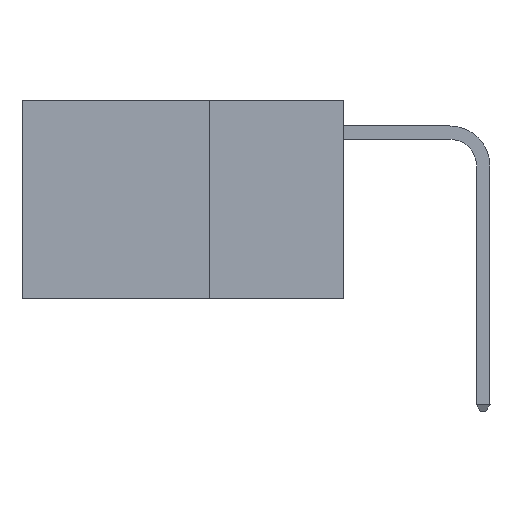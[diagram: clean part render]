
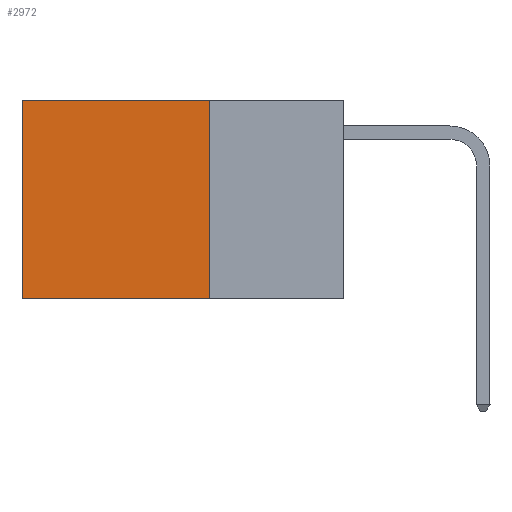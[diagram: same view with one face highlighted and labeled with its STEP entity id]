
A CAD part, left-side view. The second image highlights one B-rep face of the part: STEP entity #2972.
In plain terms, the highlighted planar face has unit normal (-1, 0, 0).
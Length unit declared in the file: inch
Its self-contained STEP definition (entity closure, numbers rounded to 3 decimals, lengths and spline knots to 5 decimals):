
#190 = ORIENTED_EDGE ( 'NONE', *, *, #12204, .T. ) ;
#809 = CARTESIAN_POINT ( 'NONE',  ( 0.2625, 0.25, 0. ) ) ;
#930 = VERTEX_POINT ( 'NONE', #4951 ) ;
#1069 = EDGE_CURVE ( 'NONE', #10929, #2018, #9868, .T. ) ;
#1940 = DIRECTION ( 'NONE',  ( 0., 0., -1. ) ) ;
#2018 = VERTEX_POINT ( 'NONE', #9913 ) ;
#2113 = EDGE_CURVE ( 'NONE', #930, #2018, #4363, .T. ) ;
#2619 = CARTESIAN_POINT ( 'NONE',  ( 0.2625, 0.25, 0. ) ) ;
#2911 = CARTESIAN_POINT ( 'NONE',  ( 0.2625, 0.25, 0. ) ) ;
#2942 = VECTOR ( 'NONE', #9457, 39.37008 ) ;
#2972 = ADVANCED_FACE ( 'NONE', ( #8832 ), #11843, .F. ) ;
#3002 = VECTOR ( 'NONE', #3671, 39.37008 ) ;
#3385 = CARTESIAN_POINT ( 'NONE',  ( 0.2625, 0.6, 0. ) ) ;
#3497 = VECTOR ( 'NONE', #6659, 39.37008 ) ;
#3577 = VERTEX_POINT ( 'NONE', #11194 ) ;
#3671 = DIRECTION ( 'NONE',  ( 0., 1., 0. ) ) ;
#3788 = ORIENTED_EDGE ( 'NONE', *, *, #10650, .F. ) ;
#4346 = EDGE_LOOP ( 'NONE', ( #7719, #10934, #3788, #190 ) ) ;
#4363 = LINE ( 'NONE', #3385, #2942 ) ;
#4508 = CARTESIAN_POINT ( 'NONE',  ( 0.2625, 0.25, -0.37 ) ) ;
#4951 = CARTESIAN_POINT ( 'NONE',  ( 0.2625, 0.6, 0. ) ) ;
#5305 = AXIS2_PLACEMENT_3D ( 'NONE', #809, #6893, #1940 ) ;
#6659 = DIRECTION ( 'NONE',  ( 0., 1., 0. ) ) ;
#6893 = DIRECTION ( 'NONE',  ( 1., 0., 0. ) ) ;
#7272 = VECTOR ( 'NONE', #9985, 39.37008 ) ;
#7719 = ORIENTED_EDGE ( 'NONE', *, *, #2113, .T. ) ;
#8642 = CARTESIAN_POINT ( 'NONE',  ( 0.2625, 0.25, -0.37 ) ) ;
#8832 = FACE_OUTER_BOUND ( 'NONE', #4346, .T. ) ;
#9457 = DIRECTION ( 'NONE',  ( 0., 0., -1. ) ) ;
#9868 = LINE ( 'NONE', #8642, #3002 ) ;
#9913 = CARTESIAN_POINT ( 'NONE',  ( 0.2625, 0.6, -0.37 ) ) ;
#9985 = DIRECTION ( 'NONE',  ( 0., 0., -1. ) ) ;
#10650 = EDGE_CURVE ( 'NONE', #3577, #10929, #10842, .T. ) ;
#10842 = LINE ( 'NONE', #2911, #7272 ) ;
#10929 = VERTEX_POINT ( 'NONE', #4508 ) ;
#10934 = ORIENTED_EDGE ( 'NONE', *, *, #1069, .F. ) ;
#11194 = CARTESIAN_POINT ( 'NONE',  ( 0.2625, 0.25, 0. ) ) ;
#11843 = PLANE ( 'NONE',  #5305 ) ;
#12204 = EDGE_CURVE ( 'NONE', #3577, #930, #12541, .T. ) ;
#12541 = LINE ( 'NONE', #2619, #3497 ) ;
